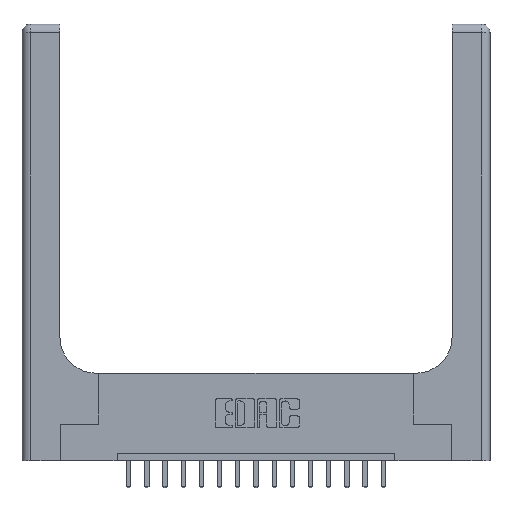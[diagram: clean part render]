
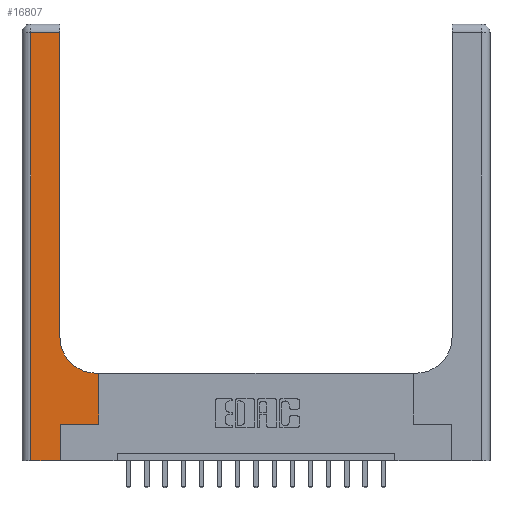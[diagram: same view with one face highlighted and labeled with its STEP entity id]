
A CAD part, top view. The second image highlights one B-rep face of the part: STEP entity #16807.
In plain terms, the highlighted planar face has unit normal (0, 0, 1).
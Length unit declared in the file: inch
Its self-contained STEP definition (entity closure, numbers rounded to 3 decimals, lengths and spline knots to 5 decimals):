
#31 = VECTOR ( 'NONE', #15345, 39.37008 ) ;
#424 = EDGE_LOOP ( 'NONE', ( #1073, #2825, #15278, #12086, #16962, #7483, #9530, #1389, #12352 ) ) ;
#1005 = LINE ( 'NONE', #5067, #17626 ) ;
#1073 = ORIENTED_EDGE ( 'NONE', *, *, #6230, .T. ) ;
#1112 = CARTESIAN_POINT ( 'NONE',  ( 0., 0., 0.37 ) ) ;
#1389 = ORIENTED_EDGE ( 'NONE', *, *, #7259, .T. ) ;
#1425 = DIRECTION ( 'NONE',  ( 0., 1., 0. ) ) ;
#1475 = CARTESIAN_POINT ( 'NONE',  ( 0.26, 0.85, 0.37 ) ) ;
#1571 = DIRECTION ( 'NONE',  ( 0., 1., 0. ) ) ;
#1677 = CARTESIAN_POINT ( 'NONE',  ( 0., 2.94, 0.37 ) ) ;
#2349 = CARTESIAN_POINT ( 'NONE',  ( 0.06, 2.94, 0.37 ) ) ;
#2396 = CIRCLE ( 'NONE', #7216, 0.25 ) ;
#2825 = ORIENTED_EDGE ( 'NONE', *, *, #15495, .T. ) ;
#3129 = VERTEX_POINT ( 'NONE', #4945 ) ;
#3411 = LINE ( 'NONE', #10678, #18270 ) ;
#3439 = CARTESIAN_POINT ( 'NONE',  ( 0.51, 0.6, 0.37 ) ) ;
#3453 = VERTEX_POINT ( 'NONE', #2349 ) ;
#3750 = DIRECTION ( 'NONE',  ( 1., 0., 0. ) ) ;
#4295 = VECTOR ( 'NONE', #1571, 39.37008 ) ;
#4403 = LINE ( 'NONE', #4501, #4295 ) ;
#4501 = CARTESIAN_POINT ( 'NONE',  ( 0.528, 0.25, 0.37 ) ) ;
#4709 = DIRECTION ( 'NONE',  ( 1., 0., 0. ) ) ;
#4902 = DIRECTION ( 'NONE',  ( 1., 0., 0. ) ) ;
#4945 = CARTESIAN_POINT ( 'NONE',  ( 0.26, 2.94, 0.37 ) ) ;
#5067 = CARTESIAN_POINT ( 'NONE',  ( 0.26, 3., 0.37 ) ) ;
#5119 = EDGE_CURVE ( 'NONE', #17388, #6844, #6598, .T. ) ;
#6088 = AXIS2_PLACEMENT_3D ( 'NONE', #16856, #8269, #9397 ) ;
#6230 = EDGE_CURVE ( 'NONE', #17949, #3129, #1005, .T. ) ;
#6417 = LINE ( 'NONE', #16315, #17699 ) ;
#6598 = LINE ( 'NONE', #1112, #16726 ) ;
#6771 = DIRECTION ( 'NONE',  ( 0., 1., 0. ) ) ;
#6844 = VERTEX_POINT ( 'NONE', #9755 ) ;
#7216 = AXIS2_PLACEMENT_3D ( 'NONE', #13684, #12257, #4902 ) ;
#7259 = EDGE_CURVE ( 'NONE', #10859, #14251, #3411, .T. ) ;
#7483 = ORIENTED_EDGE ( 'NONE', *, *, #8925, .T. ) ;
#7992 = FACE_OUTER_BOUND ( 'NONE', #424, .T. ) ;
#8169 = VECTOR ( 'NONE', #13566, 39.37008 ) ;
#8178 = LINE ( 'NONE', #14035, #31 ) ;
#8269 = DIRECTION ( 'NONE',  ( 0., 0., -1. ) ) ;
#8925 = EDGE_CURVE ( 'NONE', #15162, #15627, #6417, .T. ) ;
#9180 = DIRECTION ( 'NONE',  ( -1., 0., 0. ) ) ;
#9305 = LINE ( 'NONE', #1677, #8169 ) ;
#9397 = DIRECTION ( 'NONE',  ( -1., 0., 0. ) ) ;
#9530 = ORIENTED_EDGE ( 'NONE', *, *, #17914, .T. ) ;
#9579 = PLANE ( 'NONE',  #6088 ) ;
#9755 = CARTESIAN_POINT ( 'NONE',  ( 0.265, 0., 0.37 ) ) ;
#10029 = CARTESIAN_POINT ( 'NONE',  ( 0.528, 0.6, 0.37 ) ) ;
#10678 = CARTESIAN_POINT ( 'NONE',  ( 0.26, 0.6, 0.37 ) ) ;
#10859 = VERTEX_POINT ( 'NONE', #10029 ) ;
#11150 = LINE ( 'NONE', #14362, #17247 ) ;
#11208 = CARTESIAN_POINT ( 'NONE',  ( 0.265, 0.25, 0.37 ) ) ;
#11550 = EDGE_CURVE ( 'NONE', #14251, #17949, #2396, .T. ) ;
#12086 = ORIENTED_EDGE ( 'NONE', *, *, #5119, .T. ) ;
#12257 = DIRECTION ( 'NONE',  ( 0., 0., -1. ) ) ;
#12352 = ORIENTED_EDGE ( 'NONE', *, *, #11550, .T. ) ;
#12520 = CARTESIAN_POINT ( 'NONE',  ( 0.528, 0.25, 0.37 ) ) ;
#13566 = DIRECTION ( 'NONE',  ( -1., 0., 0. ) ) ;
#13684 = CARTESIAN_POINT ( 'NONE',  ( 0.51, 0.85, 0.37 ) ) ;
#14035 = CARTESIAN_POINT ( 'NONE',  ( 0.06, 3., 0.37 ) ) ;
#14251 = VERTEX_POINT ( 'NONE', #3439 ) ;
#14362 = CARTESIAN_POINT ( 'NONE',  ( 0.265, 0., 0.37 ) ) ;
#15162 = VERTEX_POINT ( 'NONE', #11208 ) ;
#15278 = ORIENTED_EDGE ( 'NONE', *, *, #16771, .T. ) ;
#15345 = DIRECTION ( 'NONE',  ( 0., -1., 0. ) ) ;
#15495 = EDGE_CURVE ( 'NONE', #3129, #3453, #9305, .T. ) ;
#15627 = VERTEX_POINT ( 'NONE', #12520 ) ;
#16315 = CARTESIAN_POINT ( 'NONE',  ( 0.265, 0.25, 0.37 ) ) ;
#16726 = VECTOR ( 'NONE', #3750, 39.37008 ) ;
#16727 = CARTESIAN_POINT ( 'NONE',  ( 0.06, 0., 0.37 ) ) ;
#16771 = EDGE_CURVE ( 'NONE', #3453, #17388, #8178, .T. ) ;
#16807 = ADVANCED_FACE ( 'NONE', ( #7992 ), #9579, .F. ) ;
#16856 = CARTESIAN_POINT ( 'NONE',  ( 0., 3., 0.37 ) ) ;
#16962 = ORIENTED_EDGE ( 'NONE', *, *, #17537, .T. ) ;
#17247 = VECTOR ( 'NONE', #1425, 39.37008 ) ;
#17388 = VERTEX_POINT ( 'NONE', #16727 ) ;
#17537 = EDGE_CURVE ( 'NONE', #6844, #15162, #11150, .T. ) ;
#17626 = VECTOR ( 'NONE', #6771, 39.37008 ) ;
#17699 = VECTOR ( 'NONE', #4709, 39.37008 ) ;
#17914 = EDGE_CURVE ( 'NONE', #15627, #10859, #4403, .T. ) ;
#17949 = VERTEX_POINT ( 'NONE', #1475 ) ;
#18270 = VECTOR ( 'NONE', #9180, 39.37008 ) ;
